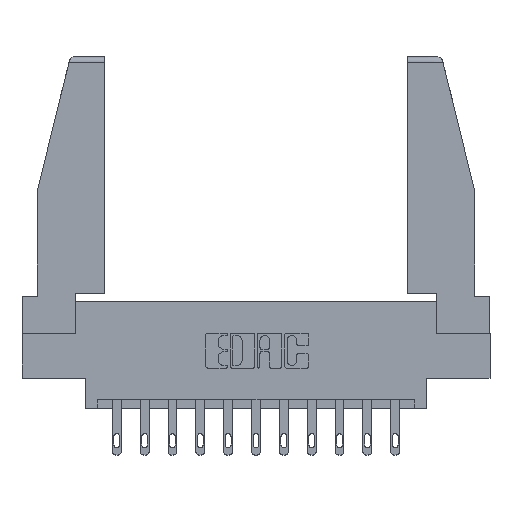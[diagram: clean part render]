
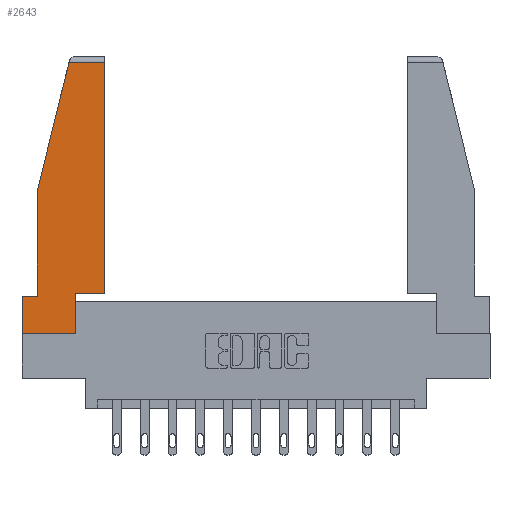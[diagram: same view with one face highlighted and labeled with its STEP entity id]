
A CAD part, top view. The second image highlights one B-rep face of the part: STEP entity #2643.
In plain terms, the highlighted planar face has unit normal (0, 0, 1).
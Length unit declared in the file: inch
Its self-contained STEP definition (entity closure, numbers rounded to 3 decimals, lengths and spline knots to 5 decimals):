
#24 = LINE ( 'NONE', #10127, #13306 ) ;
#59 = AXIS2_PLACEMENT_3D ( 'NONE', #14267, #6241, #6195 ) ;
#524 = CARTESIAN_POINT ( 'NONE',  ( 0., 0.21, 0. ) ) ;
#903 = CARTESIAN_POINT ( 'NONE',  ( 0.461, 1.52, 0. ) ) ;
#961 = EDGE_CURVE ( 'NONE', #5441, #9711, #3332, .T. ) ;
#1443 = ORIENTED_EDGE ( 'NONE', *, *, #8123, .T. ) ;
#1502 = VERTEX_POINT ( 'NONE', #4665 ) ;
#1983 = CARTESIAN_POINT ( 'NONE',  ( 0.086, 0.8, 0. ) ) ;
#2206 = VERTEX_POINT ( 'NONE', #11362 ) ;
#2380 = VERTEX_POINT ( 'NONE', #5084 ) ;
#2425 = VERTEX_POINT ( 'NONE', #10972 ) ;
#2643 = ADVANCED_FACE ( 'NONE', ( #11859 ), #8457, .T. ) ;
#3088 = DIRECTION ( 'NONE',  ( -1., 0., 0. ) ) ;
#3168 = LINE ( 'NONE', #8172, #5192 ) ;
#3332 = LINE ( 'NONE', #12390, #8322 ) ;
#3586 = VECTOR ( 'NONE', #5734, 39.37008 ) ;
#3888 = EDGE_LOOP ( 'NONE', ( #11342, #9281, #6754, #7119, #1443, #11742, #10077, #11559, #6772 ) ) ;
#4260 = CARTESIAN_POINT ( 'NONE',  ( 0., 0., 0. ) ) ;
#4433 = VERTEX_POINT ( 'NONE', #903 ) ;
#4472 = VERTEX_POINT ( 'NONE', #8235 ) ;
#4665 = CARTESIAN_POINT ( 'NONE',  ( 0., 0.21, 0. ) ) ;
#4783 = VECTOR ( 'NONE', #10368, 39.37008 ) ;
#4813 = LINE ( 'NONE', #524, #14088 ) ;
#5084 = CARTESIAN_POINT ( 'NONE',  ( 0.2636, 1.52, 0. ) ) ;
#5192 = VECTOR ( 'NONE', #10558, 39.37008 ) ;
#5342 = DIRECTION ( 'NONE',  ( 1., 0., 0. ) ) ;
#5441 = VERTEX_POINT ( 'NONE', #14150 ) ;
#5734 = DIRECTION ( 'NONE',  ( 0., 1., 0. ) ) ;
#5844 = EDGE_CURVE ( 'NONE', #2380, #2425, #8122, .T. ) ;
#6195 = DIRECTION ( 'NONE',  ( 1., 0., 0. ) ) ;
#6241 = DIRECTION ( 'NONE',  ( 0., 0., 1. ) ) ;
#6313 = DIRECTION ( 'NONE',  ( -0.239, -0.971, 0. ) ) ;
#6463 = VERTEX_POINT ( 'NONE', #9741 ) ;
#6754 = ORIENTED_EDGE ( 'NONE', *, *, #5844, .T. ) ;
#6772 = ORIENTED_EDGE ( 'NONE', *, *, #11300, .T. ) ;
#7023 = VECTOR ( 'NONE', #6313, 39.37008 ) ;
#7119 = ORIENTED_EDGE ( 'NONE', *, *, #14423, .T. ) ;
#7712 = LINE ( 'NONE', #1983, #4783 ) ;
#8123 = EDGE_CURVE ( 'NONE', #2206, #1502, #24, .T. ) ;
#8122 = LINE ( 'NONE', #12099, #7023 ) ;
#8172 = CARTESIAN_POINT ( 'NONE',  ( 0., 1.52, 0. ) ) ;
#8235 = CARTESIAN_POINT ( 'NONE',  ( 0.461, 0.223, 0. ) ) ;
#8322 = VECTOR ( 'NONE', #9057, 39.37008 ) ;
#8457 = PLANE ( 'NONE',  #59 ) ;
#9057 = DIRECTION ( 'NONE',  ( 0., 1., 0. ) ) ;
#9281 = ORIENTED_EDGE ( 'NONE', *, *, #12032, .T. ) ;
#9483 = CARTESIAN_POINT ( 'NONE',  ( 0.461, 0.223, 0. ) ) ;
#9711 = VERTEX_POINT ( 'NONE', #13501 ) ;
#9741 = CARTESIAN_POINT ( 'NONE',  ( 0., 0., 0. ) ) ;
#9970 = EDGE_CURVE ( 'NONE', #4472, #4433, #14520, .T. ) ;
#10077 = ORIENTED_EDGE ( 'NONE', *, *, #11012, .T. ) ;
#10127 = CARTESIAN_POINT ( 'NONE',  ( 0., 0.21, 0. ) ) ;
#10343 = CARTESIAN_POINT ( 'NONE',  ( 0.297, 0.223, 0. ) ) ;
#10368 = DIRECTION ( 'NONE',  ( 0., -1., 0. ) ) ;
#10558 = DIRECTION ( 'NONE',  ( -1., 0., 0. ) ) ;
#10972 = CARTESIAN_POINT ( 'NONE',  ( 0.086, 0.8, 0. ) ) ;
#11012 = EDGE_CURVE ( 'NONE', #6463, #5441, #11063, .T. ) ;
#11063 = LINE ( 'NONE', #4260, #11599 ) ;
#11236 = LINE ( 'NONE', #10343, #13562 ) ;
#11300 = EDGE_CURVE ( 'NONE', #9711, #4472, #11236, .T. ) ;
#11342 = ORIENTED_EDGE ( 'NONE', *, *, #9970, .T. ) ;
#11343 = DIRECTION ( 'NONE',  ( 1., 0., 0. ) ) ;
#11362 = CARTESIAN_POINT ( 'NONE',  ( 0.086, 0.21, 0. ) ) ;
#11559 = ORIENTED_EDGE ( 'NONE', *, *, #961, .T. ) ;
#11599 = VECTOR ( 'NONE', #5342, 39.37008 ) ;
#11742 = ORIENTED_EDGE ( 'NONE', *, *, #13097, .T. ) ;
#11859 = FACE_OUTER_BOUND ( 'NONE', #3888, .T. ) ;
#12032 = EDGE_CURVE ( 'NONE', #4433, #2380, #3168, .T. ) ;
#12099 = CARTESIAN_POINT ( 'NONE',  ( 0.271, 1.55, 0. ) ) ;
#12390 = CARTESIAN_POINT ( 'NONE',  ( 0.297, 0., 0. ) ) ;
#13097 = EDGE_CURVE ( 'NONE', #1502, #6463, #4813, .T. ) ;
#13306 = VECTOR ( 'NONE', #3088, 39.37008 ) ;
#13501 = CARTESIAN_POINT ( 'NONE',  ( 0.297, 0.223, 0. ) ) ;
#13562 = VECTOR ( 'NONE', #11343, 39.37008 ) ;
#14088 = VECTOR ( 'NONE', #14462, 39.37008 ) ;
#14150 = CARTESIAN_POINT ( 'NONE',  ( 0.297, 0., 0. ) ) ;
#14267 = CARTESIAN_POINT ( 'NONE',  ( 0., 0., 0. ) ) ;
#14423 = EDGE_CURVE ( 'NONE', #2425, #2206, #7712, .T. ) ;
#14462 = DIRECTION ( 'NONE',  ( 0., -1., 0. ) ) ;
#14520 = LINE ( 'NONE', #9483, #3586 ) ;
